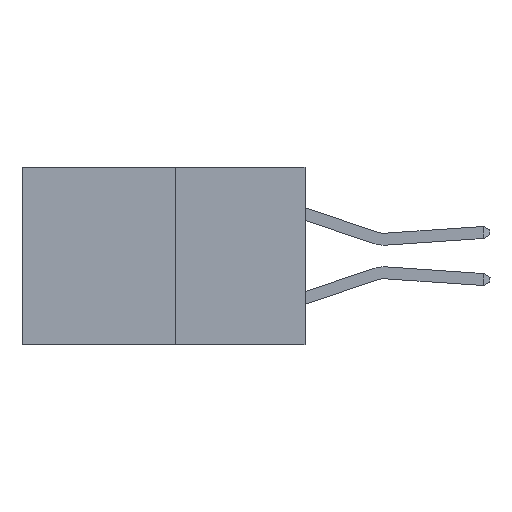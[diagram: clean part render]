
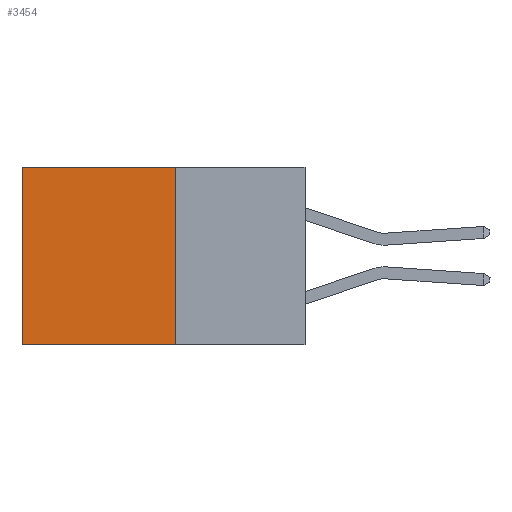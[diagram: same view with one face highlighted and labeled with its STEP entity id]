
A CAD part, left-side view. The second image highlights one B-rep face of the part: STEP entity #3454.
In plain terms, the highlighted planar face has unit normal (-1, 0, 0).
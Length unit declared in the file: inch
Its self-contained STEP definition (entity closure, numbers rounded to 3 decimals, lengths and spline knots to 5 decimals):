
#258 = CARTESIAN_POINT ( 'NONE',  ( 0.277, 0.59, -0.37 ) ) ;
#440 = VECTOR ( 'NONE', #15852, 39.37008 ) ;
#759 = CARTESIAN_POINT ( 'NONE',  ( 0.277, 0.27, 0. ) ) ;
#949 = PLANE ( 'NONE',  #19955 ) ;
#1724 = CARTESIAN_POINT ( 'NONE',  ( 0.277, 0.27, -0.37 ) ) ;
#1826 = LINE ( 'NONE', #759, #440 ) ;
#2824 = CARTESIAN_POINT ( 'NONE',  ( 0.277, 0.59, 0. ) ) ;
#2991 = EDGE_LOOP ( 'NONE', ( #14831, #10529, #18777, #12176 ) ) ;
#3397 = DIRECTION ( 'NONE',  ( 1., 0., 0. ) ) ;
#3454 = ADVANCED_FACE ( 'NONE', ( #19706 ), #949, .F. ) ;
#4023 = EDGE_CURVE ( 'NONE', #13934, #16135, #17708, .T. ) ;
#4998 = LINE ( 'NONE', #258, #9437 ) ;
#5355 = CARTESIAN_POINT ( 'NONE',  ( 0.277, 0.27, -0.37 ) ) ;
#5846 = CARTESIAN_POINT ( 'NONE',  ( 0.277, 0.27, 0. ) ) ;
#6394 = VECTOR ( 'NONE', #18231, 39.37008 ) ;
#9437 = VECTOR ( 'NONE', #11191, 39.37008 ) ;
#10529 = ORIENTED_EDGE ( 'NONE', *, *, #12039, .F. ) ;
#10840 = EDGE_CURVE ( 'NONE', #13018, #14365, #4998, .T. ) ;
#11191 = DIRECTION ( 'NONE',  ( 0., 0., -1. ) ) ;
#12039 = EDGE_CURVE ( 'NONE', #16135, #14365, #24497, .T. ) ;
#12176 = ORIENTED_EDGE ( 'NONE', *, *, #16862, .T. ) ;
#13018 = VERTEX_POINT ( 'NONE', #2824 ) ;
#13934 = VERTEX_POINT ( 'NONE', #5846 ) ;
#14365 = VERTEX_POINT ( 'NONE', #23873 ) ;
#14640 = CARTESIAN_POINT ( 'NONE',  ( 0.277, 0.27, -0.37 ) ) ;
#14831 = ORIENTED_EDGE ( 'NONE', *, *, #10840, .T. ) ;
#15852 = DIRECTION ( 'NONE',  ( 0., 1., 0. ) ) ;
#16135 = VERTEX_POINT ( 'NONE', #25341 ) ;
#16862 = EDGE_CURVE ( 'NONE', #13934, #13018, #1826, .T. ) ;
#17708 = LINE ( 'NONE', #5355, #6394 ) ;
#18231 = DIRECTION ( 'NONE',  ( 0., 0., -1. ) ) ;
#18777 = ORIENTED_EDGE ( 'NONE', *, *, #4023, .F. ) ;
#18959 = VECTOR ( 'NONE', #25082, 39.37008 ) ;
#19706 = FACE_OUTER_BOUND ( 'NONE', #2991, .T. ) ;
#19937 = DIRECTION ( 'NONE',  ( 0., 0., -1. ) ) ;
#19955 = AXIS2_PLACEMENT_3D ( 'NONE', #14640, #3397, #19937 ) ;
#23873 = CARTESIAN_POINT ( 'NONE',  ( 0.277, 0.59, -0.37 ) ) ;
#24497 = LINE ( 'NONE', #1724, #18959 ) ;
#25082 = DIRECTION ( 'NONE',  ( 0., 1., 0. ) ) ;
#25341 = CARTESIAN_POINT ( 'NONE',  ( 0.277, 0.27, -0.37 ) ) ;
